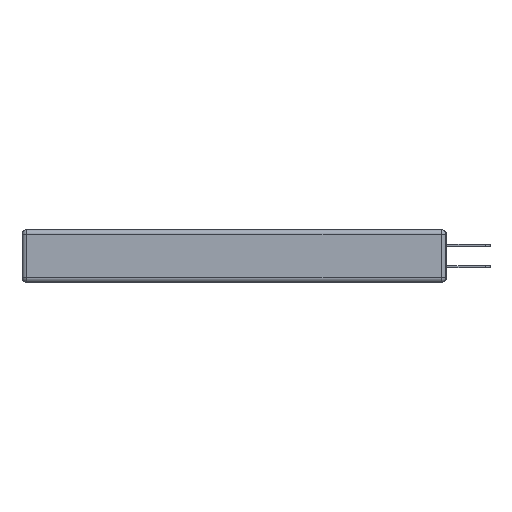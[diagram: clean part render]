
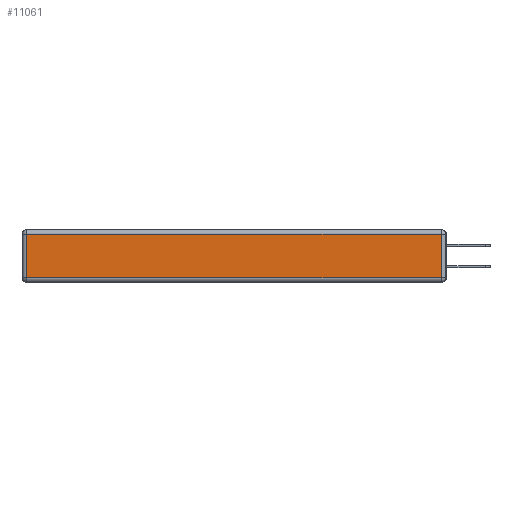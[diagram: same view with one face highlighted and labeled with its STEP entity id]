
A CAD part, left-side view. The second image highlights one B-rep face of the part: STEP entity #11061.
In plain terms, the highlighted planar face has unit normal (-1, 0, 0).
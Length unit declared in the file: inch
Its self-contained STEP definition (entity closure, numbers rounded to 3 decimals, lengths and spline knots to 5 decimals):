
#316 = DIRECTION ( 'NONE',  ( 0., -1., 0. ) ) ;
#745 = VECTOR ( 'NONE', #16712, 39.37008 ) ;
#1299 = FACE_OUTER_BOUND ( 'NONE', #10657, .T. ) ;
#1539 = CARTESIAN_POINT ( 'NONE',  ( 0., 0., -0.343 ) ) ;
#2179 = ORIENTED_EDGE ( 'NONE', *, *, #13602, .T. ) ;
#3412 = VECTOR ( 'NONE', #15252, 39.37008 ) ;
#3813 = PLANE ( 'NONE',  #20902 ) ;
#4019 = VERTEX_POINT ( 'NONE', #24242 ) ;
#4031 = VECTOR ( 'NONE', #316, 39.37008 ) ;
#5315 = CARTESIAN_POINT ( 'NONE',  ( 0., 2.72, -0.03 ) ) ;
#5319 = LINE ( 'NONE', #25532, #22546 ) ;
#5569 = DIRECTION ( 'NONE',  ( 0., 0., 1. ) ) ;
#6118 = LINE ( 'NONE', #22571, #4031 ) ;
#7667 = ORIENTED_EDGE ( 'NONE', *, *, #27436, .T. ) ;
#8077 = LINE ( 'NONE', #21120, #745 ) ;
#8443 = EDGE_CURVE ( 'NONE', #15747, #18050, #8077, .T. ) ;
#10657 = EDGE_LOOP ( 'NONE', ( #19628, #7667, #2179, #15522 ) ) ;
#11061 = ADVANCED_FACE ( 'NONE', ( #1299 ), #3813, .T. ) ;
#11789 = LINE ( 'NONE', #13108, #3412 ) ;
#13108 = CARTESIAN_POINT ( 'NONE',  ( 0., 0.03, -0.343 ) ) ;
#13602 = EDGE_CURVE ( 'NONE', #4019, #15747, #5319, .T. ) ;
#15252 = DIRECTION ( 'NONE',  ( 0., 0., 1. ) ) ;
#15522 = ORIENTED_EDGE ( 'NONE', *, *, #8443, .T. ) ;
#15747 = VERTEX_POINT ( 'NONE', #5315 ) ;
#16122 = VERTEX_POINT ( 'NONE', #26070 ) ;
#16712 = DIRECTION ( 'NONE',  ( 0., 0., -1. ) ) ;
#17400 = EDGE_CURVE ( 'NONE', #18050, #16122, #6118, .T. ) ;
#18050 = VERTEX_POINT ( 'NONE', #19422 ) ;
#19103 = DIRECTION ( 'NONE',  ( -1., 0., 0. ) ) ;
#19422 = CARTESIAN_POINT ( 'NONE',  ( 0., 2.72, -0.313 ) ) ;
#19628 = ORIENTED_EDGE ( 'NONE', *, *, #17400, .T. ) ;
#20902 = AXIS2_PLACEMENT_3D ( 'NONE', #1539, #19103, #5569 ) ;
#21120 = CARTESIAN_POINT ( 'NONE',  ( 0., 2.72, -0.343 ) ) ;
#21197 = DIRECTION ( 'NONE',  ( 0., 1., 0. ) ) ;
#22546 = VECTOR ( 'NONE', #21197, 39.37008 ) ;
#22571 = CARTESIAN_POINT ( 'NONE',  ( 0., 0., -0.313 ) ) ;
#24242 = CARTESIAN_POINT ( 'NONE',  ( 0., 0.03, -0.03 ) ) ;
#25532 = CARTESIAN_POINT ( 'NONE',  ( 0., 2.75, -0.03 ) ) ;
#26070 = CARTESIAN_POINT ( 'NONE',  ( 0., 0.03, -0.313 ) ) ;
#27436 = EDGE_CURVE ( 'NONE', #16122, #4019, #11789, .T. ) ;
